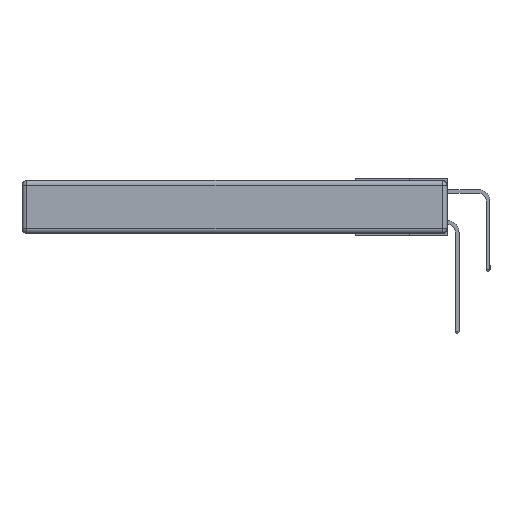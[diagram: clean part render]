
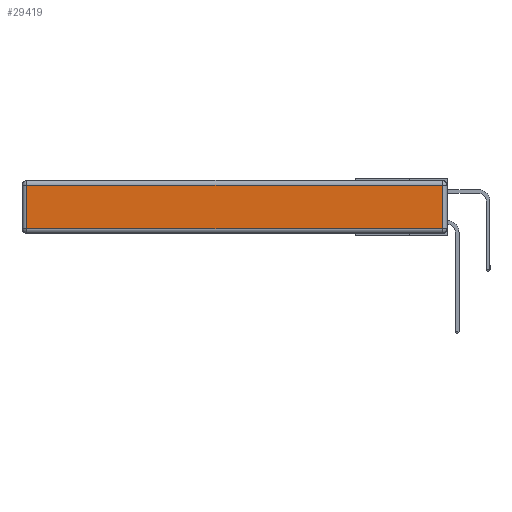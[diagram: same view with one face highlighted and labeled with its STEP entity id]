
A CAD part, left-side view. The second image highlights one B-rep face of the part: STEP entity #29419.
In plain terms, the highlighted planar face has unit normal (-1, 0, 0).
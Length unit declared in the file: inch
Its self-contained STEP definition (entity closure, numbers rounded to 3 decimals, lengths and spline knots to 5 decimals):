
#1510 = VERTEX_POINT ( 'NONE', #31216 ) ;
#3782 = VECTOR ( 'NONE', #20849, 39.37008 ) ;
#3789 = ORIENTED_EDGE ( 'NONE', *, *, #11223, .T. ) ;
#3873 = DIRECTION ( 'NONE',  ( 0., 1., 0. ) ) ;
#4239 = VECTOR ( 'NONE', #3873, 39.37008 ) ;
#4685 = ORIENTED_EDGE ( 'NONE', *, *, #17729, .T. ) ;
#7182 = ORIENTED_EDGE ( 'NONE', *, *, #17510, .T. ) ;
#7222 = LINE ( 'NONE', #13346, #3782 ) ;
#8398 = CARTESIAN_POINT ( 'NONE',  ( 0., 0.03, -0.03 ) ) ;
#11223 = EDGE_CURVE ( 'NONE', #18736, #1510, #17370, .T. ) ;
#11434 = VECTOR ( 'NONE', #28618, 39.37008 ) ;
#12725 = CARTESIAN_POINT ( 'NONE',  ( 0., 0.03, -0.313 ) ) ;
#13346 = CARTESIAN_POINT ( 'NONE',  ( 0., 0., -0.313 ) ) ;
#13771 = LINE ( 'NONE', #28511, #11434 ) ;
#15191 = PLANE ( 'NONE',  #31657 ) ;
#15900 = VERTEX_POINT ( 'NONE', #12725 ) ;
#17103 = DIRECTION ( 'NONE',  ( 0., 0., -1. ) ) ;
#17370 = LINE ( 'NONE', #26938, #4239 ) ;
#17510 = EDGE_CURVE ( 'NONE', #1510, #24516, #29608, .T. ) ;
#17729 = EDGE_CURVE ( 'NONE', #15900, #18736, #13771, .T. ) ;
#18520 = EDGE_LOOP ( 'NONE', ( #21914, #4685, #3789, #7182 ) ) ;
#18736 = VERTEX_POINT ( 'NONE', #8398 ) ;
#20849 = DIRECTION ( 'NONE',  ( 0., -1., 0. ) ) ;
#21914 = ORIENTED_EDGE ( 'NONE', *, *, #28346, .T. ) ;
#22990 = VECTOR ( 'NONE', #17103, 39.37008 ) ;
#23448 = DIRECTION ( 'NONE',  ( 0., 0., 1. ) ) ;
#24516 = VERTEX_POINT ( 'NONE', #31393 ) ;
#26021 = CARTESIAN_POINT ( 'NONE',  ( 0., 0., -0.343 ) ) ;
#26938 = CARTESIAN_POINT ( 'NONE',  ( 0., 2.75, -0.03 ) ) ;
#28317 = DIRECTION ( 'NONE',  ( -1., 0., 0. ) ) ;
#28346 = EDGE_CURVE ( 'NONE', #24516, #15900, #7222, .T. ) ;
#28511 = CARTESIAN_POINT ( 'NONE',  ( 0., 0.03, -0.343 ) ) ;
#28618 = DIRECTION ( 'NONE',  ( 0., 0., 1. ) ) ;
#29419 = ADVANCED_FACE ( 'NONE', ( #29578 ), #15191, .T. ) ;
#29578 = FACE_OUTER_BOUND ( 'NONE', #18520, .T. ) ;
#29608 = LINE ( 'NONE', #29628, #22990 ) ;
#29628 = CARTESIAN_POINT ( 'NONE',  ( 0., 2.72, -0.343 ) ) ;
#31216 = CARTESIAN_POINT ( 'NONE',  ( 0., 2.72, -0.03 ) ) ;
#31393 = CARTESIAN_POINT ( 'NONE',  ( 0., 2.72, -0.313 ) ) ;
#31657 = AXIS2_PLACEMENT_3D ( 'NONE', #26021, #28317, #23448 ) ;
